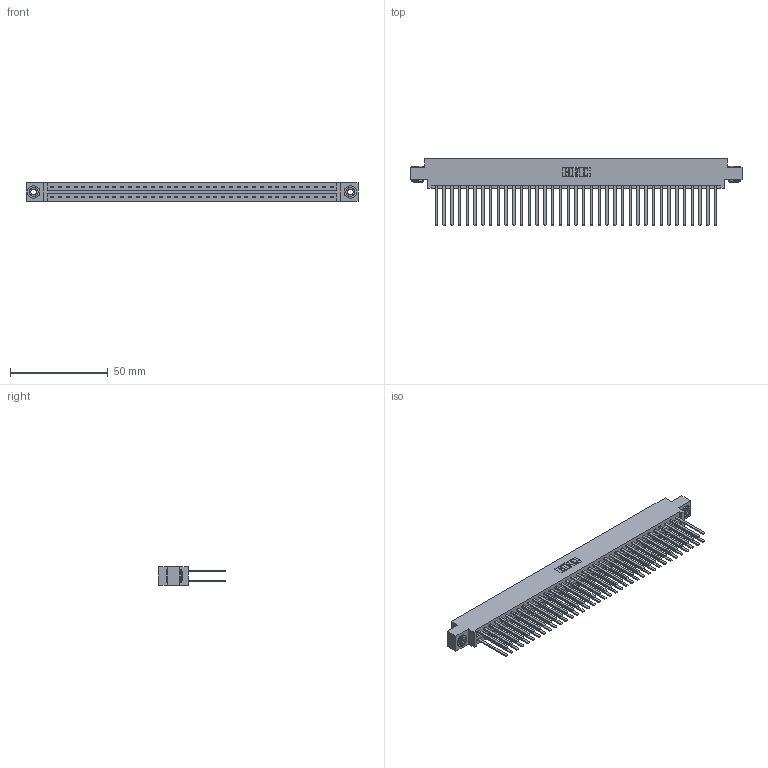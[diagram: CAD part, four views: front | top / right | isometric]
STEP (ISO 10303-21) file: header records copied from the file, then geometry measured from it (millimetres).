
FILE_DESCRIPTION (( 'STEP AP203' ), '1' );
FILE_NAME ('387-074-544-803.STEP', '2019-10-22T02:04:01', ( '' ), ( '' ), 'SwSTEP 2.0', 'SolidWorks 2016', '' );
FILE_SCHEMA (( 'CONFIG_CONTROL_DESIGN' ));
Length unit declared in the file: inch
Products named in the file (4): 387-074-544-803; 345-250-002_345-250-002-102; 345-292-001_345-293-144; 337 Part_0.170 Offset - 0.156 Dia-TH
Assembly tree (77 placements, depth 2):
  387-074-544-803
    337 Part_0.170 Offset - 0.156 Dia-TH
    345-292-001_345-293-144  x74
    345-250-002_345-250-002-102  x2
Bounding box: 169.62 x 34.3 x 9.4 mm (x, y, z)
Volume: 18748.7 mm3; surface area: 24867.8 mm2
Topology: 77 solids, 77 shells, 3708 faces, 10981 edges, 7218 vertices
Faces by surface type: plane 2600, cylinder 1100, cone 8
Entity records: 29932 total; most frequent: CARTESIAN_POINT 5021, ORIENTED_EDGE 4950, DIRECTION 4309, EDGE_CURVE 2475, VECTOR 2327, LINE 2327, VERTEX_POINT 1646, AXIS2_PLACEMENT_3D 991
